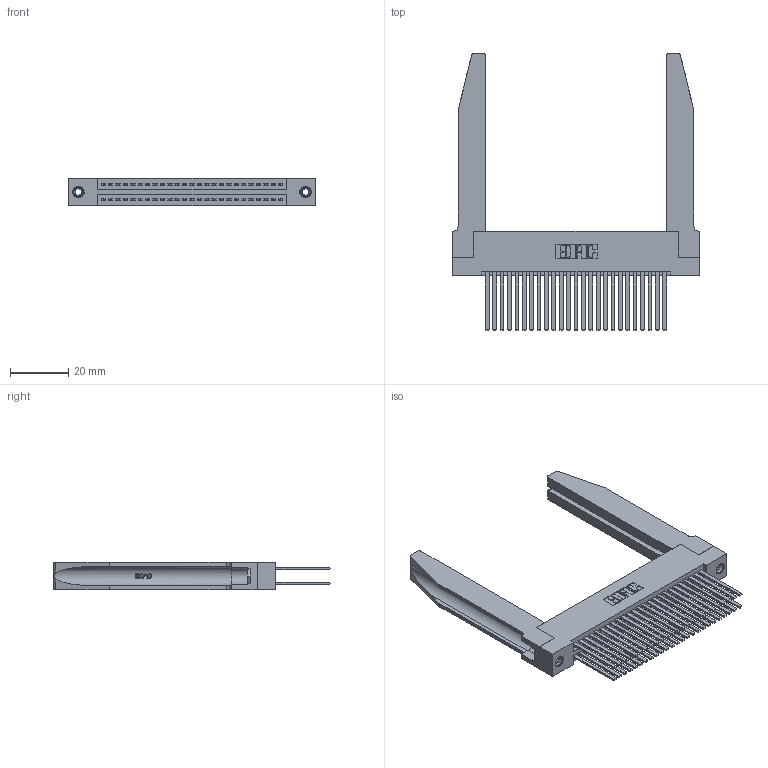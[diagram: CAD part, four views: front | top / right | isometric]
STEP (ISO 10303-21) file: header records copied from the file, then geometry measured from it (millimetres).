
FILE_DESCRIPTION (( 'STEP AP203' ), '1' );
FILE_NAME ('345-050-544-278.STEP', '2019-10-29T12:35:21', ( '' ), ( '' ), 'SwSTEP 2.0', 'SolidWorks 2016', '' );
FILE_SCHEMA (( 'CONFIG_CONTROL_DESIGN' ));
Length unit declared in the file: inch
Products named in the file (5): 345 Part_Flush Mounting Lugs - 0.156 Dia-TH; 345-050-544-278; 345-250-001_345-250-001-102; 345-220-078_345-220-078; 345-292-001_345-293-144
Assembly tree (55 placements, depth 2):
  345-050-544-278
    345 Part_Flush Mounting Lugs - 0.156 Dia-TH
    345-292-001_345-293-144  x50
    345-250-001_345-250-001-102  x2
    345-220-078_345-220-078  x2
Bounding box: 84.73 x 94.92 x 9.4 mm (x, y, z)
Volume: 16544.7 mm3; surface area: 21533.4 mm2
Topology: 55 solids, 55 shells, 2560 faces, 7499 edges, 4922 vertices
Faces by surface type: plane 1672, cylinder 836, bspline 36, cone 12, torus 4
Entity records: 26460 total; most frequent: CARTESIAN_POINT 5367, ORIENTED_EDGE 4198, DIRECTION 3745, EDGE_CURVE 2099, LINE 1777, VECTOR 1777, VERTEX_POINT 1392, AXIS2_PLACEMENT_3D 984
